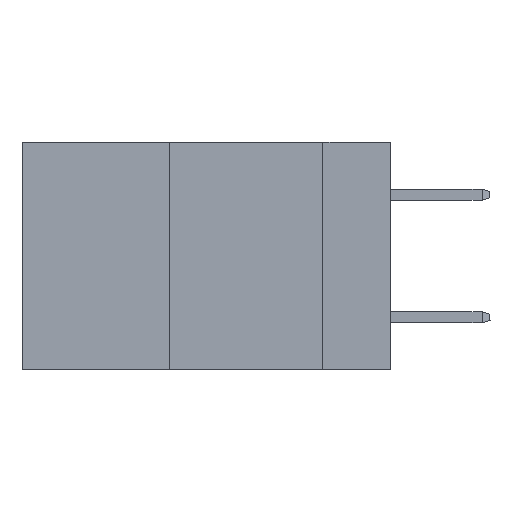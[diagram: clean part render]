
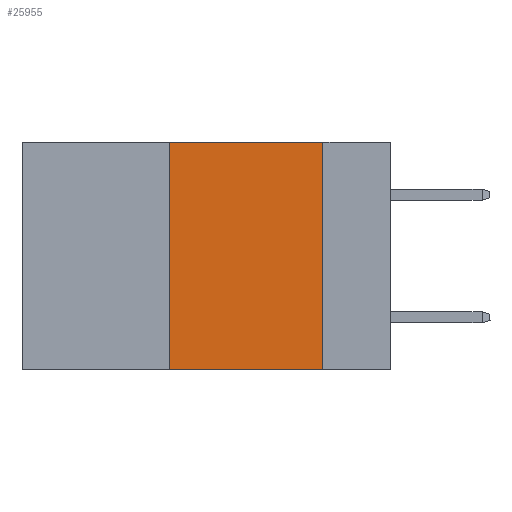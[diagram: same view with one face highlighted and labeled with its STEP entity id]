
A CAD part, left-side view. The second image highlights one B-rep face of the part: STEP entity #25955.
In plain terms, the highlighted planar face has unit normal (-1, 0, 0).
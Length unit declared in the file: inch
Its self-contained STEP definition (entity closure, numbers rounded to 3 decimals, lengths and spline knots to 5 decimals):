
#212 = LINE ( 'NONE', #24128, #27453 ) ;
#664 = VECTOR ( 'NONE', #10381, 39.37008 ) ;
#780 = CARTESIAN_POINT ( 'NONE',  ( 0., 0.11, -0.37 ) ) ;
#1162 = ORIENTED_EDGE ( 'NONE', *, *, #3971, .F. ) ;
#1607 = DIRECTION ( 'NONE',  ( 0., 0., -1. ) ) ;
#1784 = EDGE_CURVE ( 'NONE', #7112, #17473, #15764, .T. ) ;
#1926 = CARTESIAN_POINT ( 'NONE',  ( 0., 0.11, 0. ) ) ;
#1941 = ORIENTED_EDGE ( 'NONE', *, *, #7837, .F. ) ;
#2167 = VERTEX_POINT ( 'NONE', #3897 ) ;
#3157 = ORIENTED_EDGE ( 'NONE', *, *, #1784, .F. ) ;
#3175 = VECTOR ( 'NONE', #10884, 39.37008 ) ;
#3839 = LINE ( 'NONE', #16967, #3175 ) ;
#3897 = CARTESIAN_POINT ( 'NONE',  ( 0., 0.36, -0.37 ) ) ;
#3971 = EDGE_CURVE ( 'NONE', #17473, #6433, #21390, .T. ) ;
#5818 = EDGE_CURVE ( 'NONE', #2167, #6433, #212, .T. ) ;
#6408 = EDGE_LOOP ( 'NONE', ( #1162, #3157, #1941, #14711 ) ) ;
#6433 = VERTEX_POINT ( 'NONE', #780 ) ;
#7112 = VERTEX_POINT ( 'NONE', #10439 ) ;
#7837 = EDGE_CURVE ( 'NONE', #2167, #7112, #3839, .T. ) ;
#10381 = DIRECTION ( 'NONE',  ( 0., -1., 0. ) ) ;
#10439 = CARTESIAN_POINT ( 'NONE',  ( 0., 0.36, 0. ) ) ;
#10884 = DIRECTION ( 'NONE',  ( 0., 0., 1. ) ) ;
#12154 = CARTESIAN_POINT ( 'NONE',  ( 0., 0.11, 0. ) ) ;
#12269 = FACE_OUTER_BOUND ( 'NONE', #6408, .T. ) ;
#13529 = AXIS2_PLACEMENT_3D ( 'NONE', #26955, #16499, #1607 ) ;
#13902 = PLANE ( 'NONE',  #13529 ) ;
#14520 = DIRECTION ( 'NONE',  ( 0., 0., -1. ) ) ;
#14711 = ORIENTED_EDGE ( 'NONE', *, *, #5818, .T. ) ;
#15764 = LINE ( 'NONE', #20043, #664 ) ;
#16499 = DIRECTION ( 'NONE',  ( 1., 0., 0. ) ) ;
#16967 = CARTESIAN_POINT ( 'NONE',  ( 0., 0.36, 0. ) ) ;
#17473 = VERTEX_POINT ( 'NONE', #1926 ) ;
#17707 = VECTOR ( 'NONE', #14520, 39.37008 ) ;
#20043 = CARTESIAN_POINT ( 'NONE',  ( 0., 0.6, 0. ) ) ;
#21390 = LINE ( 'NONE', #12154, #17707 ) ;
#24128 = CARTESIAN_POINT ( 'NONE',  ( 0., 0.6, -0.37 ) ) ;
#24489 = DIRECTION ( 'NONE',  ( 0., -1., 0. ) ) ;
#25955 = ADVANCED_FACE ( 'NONE', ( #12269 ), #13902, .F. ) ;
#26955 = CARTESIAN_POINT ( 'NONE',  ( 0., 0.6, 0. ) ) ;
#27453 = VECTOR ( 'NONE', #24489, 39.37008 ) ;
